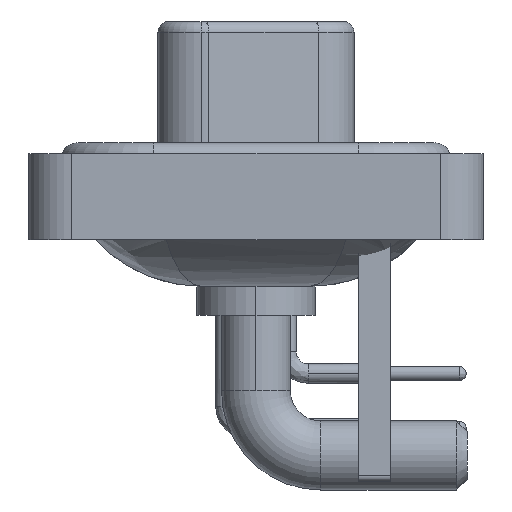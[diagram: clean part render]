
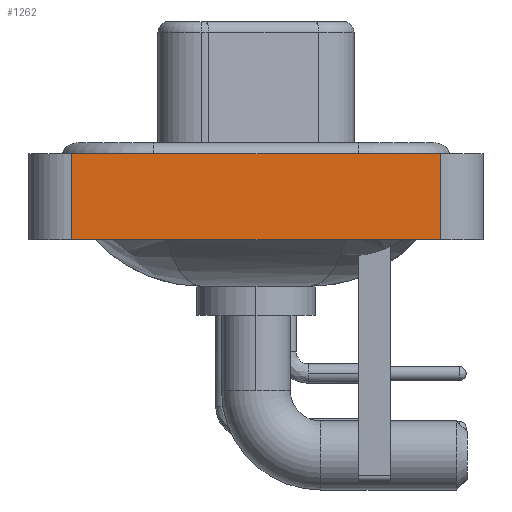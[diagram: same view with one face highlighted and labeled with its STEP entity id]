
A CAD part, left-side view. The second image highlights one B-rep face of the part: STEP entity #1262.
In plain terms, the highlighted planar face has unit normal (-1, 0, 0).
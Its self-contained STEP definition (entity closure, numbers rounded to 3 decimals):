
#295 = EDGE_CURVE ( 'NONE', #8400, #25303, #11201, .T. ) ;
#349 = DIRECTION ( 'NONE',  ( 0., 0., 1. ) ) ;
#1262 = ADVANCED_FACE ( 'NONE', ( #3519 ), #23913, .T. ) ;
#1313 = DIRECTION ( 'NONE',  ( 0., -1., 0. ) ) ;
#1429 = ORIENTED_EDGE ( 'NONE', *, *, #22511, .T. ) ;
#2344 = LINE ( 'NONE', #10633, #17114 ) ;
#2409 = CARTESIAN_POINT ( 'NONE',  ( -7.35, -8.55, 0.4 ) ) ;
#2782 = CARTESIAN_POINT ( 'NONE',  ( -7.35, -8.55, -3.6 ) ) ;
#3155 = CARTESIAN_POINT ( 'NONE',  ( -7.35, 8.55, 0.4 ) ) ;
#3519 = FACE_OUTER_BOUND ( 'NONE', #8892, .T. ) ;
#5149 = CARTESIAN_POINT ( 'NONE',  ( -7.35, 8.55, -3.6 ) ) ;
#5275 = DIRECTION ( 'NONE',  ( -1., 0., 0. ) ) ;
#7320 = CARTESIAN_POINT ( 'NONE',  ( -7.35, -8.55, -3.6 ) ) ;
#7795 = CARTESIAN_POINT ( 'NONE',  ( -7.35, 8.55, -3.6 ) ) ;
#8400 = VERTEX_POINT ( 'NONE', #5149 ) ;
#8454 = VECTOR ( 'NONE', #10744, 1000. ) ;
#8853 = VECTOR ( 'NONE', #1313, 1000. ) ;
#8892 = EDGE_LOOP ( 'NONE', ( #1429, #10895, #13172, #19646 ) ) ;
#9483 = DIRECTION ( 'NONE',  ( 0., 0., 1. ) ) ;
#10633 = CARTESIAN_POINT ( 'NONE',  ( -7.35, -8.55, 0.4 ) ) ;
#10744 = DIRECTION ( 'NONE',  ( 0., 0., 1. ) ) ;
#10895 = ORIENTED_EDGE ( 'NONE', *, *, #24234, .F. ) ;
#11201 = LINE ( 'NONE', #23598, #8853 ) ;
#13172 = ORIENTED_EDGE ( 'NONE', *, *, #19132, .F. ) ;
#16906 = LINE ( 'NONE', #2782, #18903 ) ;
#17114 = VECTOR ( 'NONE', #18956, 1000. ) ;
#18903 = VECTOR ( 'NONE', #349, 1000. ) ;
#18956 = DIRECTION ( 'NONE',  ( 0., -1., 0. ) ) ;
#19132 = EDGE_CURVE ( 'NONE', #8400, #25963, #20718, .T. ) ;
#19646 = ORIENTED_EDGE ( 'NONE', *, *, #295, .T. ) ;
#20718 = LINE ( 'NONE', #7795, #8454 ) ;
#21875 = CARTESIAN_POINT ( 'NONE',  ( -7.35, -8.55, -3.6 ) ) ;
#22033 = VERTEX_POINT ( 'NONE', #2409 ) ;
#22511 = EDGE_CURVE ( 'NONE', #25303, #22033, #16906, .T. ) ;
#23598 = CARTESIAN_POINT ( 'NONE',  ( -7.35, -8.55, -3.6 ) ) ;
#23913 = PLANE ( 'NONE',  #25438 ) ;
#24234 = EDGE_CURVE ( 'NONE', #25963, #22033, #2344, .T. ) ;
#25303 = VERTEX_POINT ( 'NONE', #7320 ) ;
#25438 = AXIS2_PLACEMENT_3D ( 'NONE', #21875, #5275, #9483 ) ;
#25963 = VERTEX_POINT ( 'NONE', #3155 ) ;
